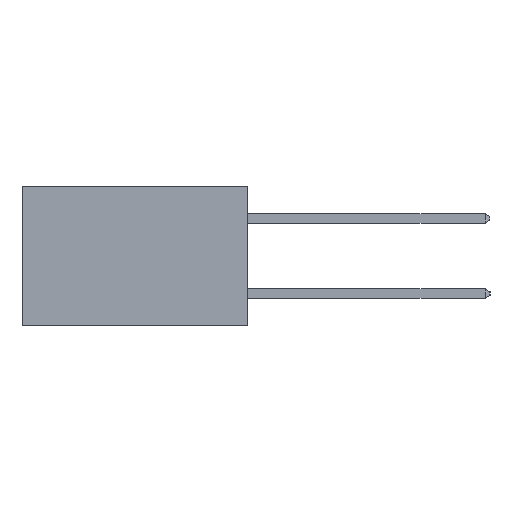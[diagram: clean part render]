
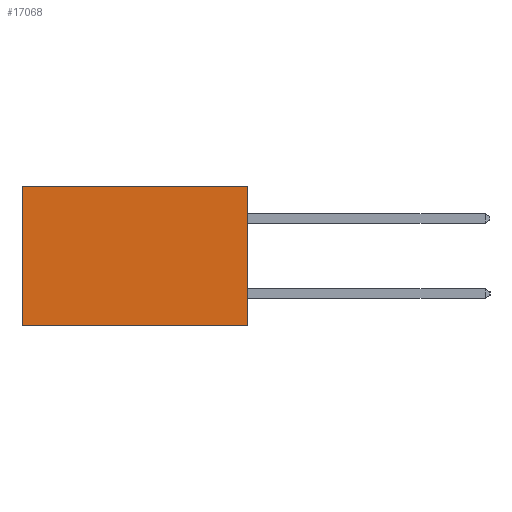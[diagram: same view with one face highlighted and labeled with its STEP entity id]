
A CAD part, left-side view. The second image highlights one B-rep face of the part: STEP entity #17068.
In plain terms, the highlighted planar face has unit normal (-1, 0, 0).
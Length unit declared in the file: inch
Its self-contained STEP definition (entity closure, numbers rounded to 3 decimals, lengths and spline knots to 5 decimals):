
#1213 = LINE ( 'NONE', #10441, #17066 ) ;
#2053 = CARTESIAN_POINT ( 'NONE',  ( 0.2615, 0., 0. ) ) ;
#3089 = ORIENTED_EDGE ( 'NONE', *, *, #23235, .T. ) ;
#3957 = AXIS2_PLACEMENT_3D ( 'NONE', #4727, #20418, #8736 ) ;
#4727 = CARTESIAN_POINT ( 'NONE',  ( 0.2615, 0., -0.37 ) ) ;
#6504 = CARTESIAN_POINT ( 'NONE',  ( 0.2615, 0., 0. ) ) ;
#7059 = CARTESIAN_POINT ( 'NONE',  ( 0.2615, 0.6, 0. ) ) ;
#7072 = VERTEX_POINT ( 'NONE', #2053 ) ;
#7847 = LINE ( 'NONE', #6504, #23304 ) ;
#8069 = FACE_OUTER_BOUND ( 'NONE', #20621, .T. ) ;
#8488 = EDGE_CURVE ( 'NONE', #7072, #17792, #7847, .T. ) ;
#8736 = DIRECTION ( 'NONE',  ( 0., 0., -1. ) ) ;
#9204 = CARTESIAN_POINT ( 'NONE',  ( 0.2615, 0., -0.37 ) ) ;
#9930 = EDGE_CURVE ( 'NONE', #18464, #19906, #1213, .T. ) ;
#10304 = LINE ( 'NONE', #19879, #20062 ) ;
#10441 = CARTESIAN_POINT ( 'NONE',  ( 0.2615, 0., -0.37 ) ) ;
#13472 = CARTESIAN_POINT ( 'NONE',  ( 0.2615, 0.6, -0.37 ) ) ;
#14238 = LINE ( 'NONE', #13472, #20020 ) ;
#14296 = DIRECTION ( 'NONE',  ( 0., 1., 0. ) ) ;
#15842 = EDGE_CURVE ( 'NONE', #7072, #18464, #10304, .T. ) ;
#16345 = CARTESIAN_POINT ( 'NONE',  ( 0.2615, 0.6, -0.37 ) ) ;
#16977 = ORIENTED_EDGE ( 'NONE', *, *, #15842, .F. ) ;
#17066 = VECTOR ( 'NONE', #14296, 39.37008 ) ;
#17068 = ADVANCED_FACE ( 'NONE', ( #8069 ), #18536, .F. ) ;
#17792 = VERTEX_POINT ( 'NONE', #7059 ) ;
#18321 = DIRECTION ( 'NONE',  ( 0., 1., 0. ) ) ;
#18464 = VERTEX_POINT ( 'NONE', #9204 ) ;
#18536 = PLANE ( 'NONE',  #3957 ) ;
#19879 = CARTESIAN_POINT ( 'NONE',  ( 0.2615, 0., -0.37 ) ) ;
#19906 = VERTEX_POINT ( 'NONE', #16345 ) ;
#20020 = VECTOR ( 'NONE', #24904, 39.37008 ) ;
#20037 = ORIENTED_EDGE ( 'NONE', *, *, #8488, .T. ) ;
#20062 = VECTOR ( 'NONE', #21749, 39.37008 ) ;
#20418 = DIRECTION ( 'NONE',  ( 1., 0., 0. ) ) ;
#20621 = EDGE_LOOP ( 'NONE', ( #3089, #23077, #16977, #20037 ) ) ;
#21749 = DIRECTION ( 'NONE',  ( 0., 0., -1. ) ) ;
#23077 = ORIENTED_EDGE ( 'NONE', *, *, #9930, .F. ) ;
#23235 = EDGE_CURVE ( 'NONE', #17792, #19906, #14238, .T. ) ;
#23304 = VECTOR ( 'NONE', #18321, 39.37008 ) ;
#24904 = DIRECTION ( 'NONE',  ( 0., 0., -1. ) ) ;
